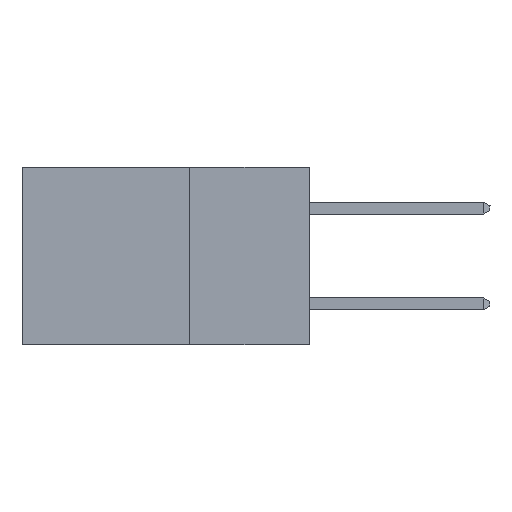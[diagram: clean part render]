
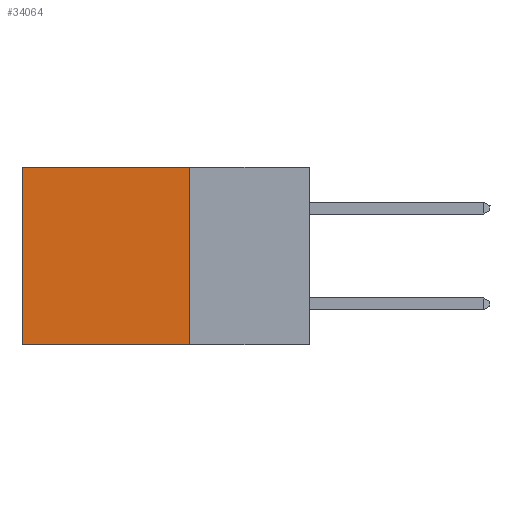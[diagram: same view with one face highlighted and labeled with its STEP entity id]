
A CAD part, left-side view. The second image highlights one B-rep face of the part: STEP entity #34064.
In plain terms, the highlighted planar face has unit normal (-1, 0, 0).
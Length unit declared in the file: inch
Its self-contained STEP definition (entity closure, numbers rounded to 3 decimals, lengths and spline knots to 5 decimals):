
#1798 = CARTESIAN_POINT ( 'NONE',  ( 0.2875, 0.25, 0. ) ) ;
#3241 = DIRECTION ( 'NONE',  ( 0., 0., -1. ) ) ;
#6987 = CARTESIAN_POINT ( 'NONE',  ( 0.2875, 0.25, -0.37 ) ) ;
#7099 = FACE_OUTER_BOUND ( 'NONE', #17099, .T. ) ;
#7116 = AXIS2_PLACEMENT_3D ( 'NONE', #1798, #23718, #32260 ) ;
#7215 = EDGE_CURVE ( 'NONE', #31215, #29491, #27271, .T. ) ;
#7290 = VECTOR ( 'NONE', #34912, 39.37008 ) ;
#8264 = LINE ( 'NONE', #27615, #22434 ) ;
#8357 = CARTESIAN_POINT ( 'NONE',  ( 0.2875, 0.6, 0. ) ) ;
#9704 = DIRECTION ( 'NONE',  ( 0., 0., -1. ) ) ;
#10205 = PLANE ( 'NONE',  #7116 ) ;
#10674 = CARTESIAN_POINT ( 'NONE',  ( 0.2875, 0.25, 0. ) ) ;
#10877 = CARTESIAN_POINT ( 'NONE',  ( 0.2875, 0.6, 0. ) ) ;
#11370 = LINE ( 'NONE', #20464, #34290 ) ;
#15477 = ORIENTED_EDGE ( 'NONE', *, *, #28930, .T. ) ;
#16179 = CARTESIAN_POINT ( 'NONE',  ( 0.2875, 0.6, -0.37 ) ) ;
#17099 = EDGE_LOOP ( 'NONE', ( #15477, #25730, #31753, #21285 ) ) ;
#18886 = EDGE_CURVE ( 'NONE', #31807, #20198, #8264, .T. ) ;
#20198 = VERTEX_POINT ( 'NONE', #16179 ) ;
#20464 = CARTESIAN_POINT ( 'NONE',  ( 0.2875, 0.25, 0. ) ) ;
#21285 = ORIENTED_EDGE ( 'NONE', *, *, #7215, .T. ) ;
#22434 = VECTOR ( 'NONE', #27258, 39.37008 ) ;
#22590 = LINE ( 'NONE', #8357, #22680 ) ;
#22680 = VECTOR ( 'NONE', #3241, 39.37008 ) ;
#23718 = DIRECTION ( 'NONE',  ( 1., 0., 0. ) ) ;
#24991 = CARTESIAN_POINT ( 'NONE',  ( 0.2875, 0.25, 0. ) ) ;
#25730 = ORIENTED_EDGE ( 'NONE', *, *, #18886, .F. ) ;
#27258 = DIRECTION ( 'NONE',  ( 0., 1., 0. ) ) ;
#27271 = LINE ( 'NONE', #10674, #7290 ) ;
#27615 = CARTESIAN_POINT ( 'NONE',  ( 0.2875, 0.25, -0.37 ) ) ;
#28154 = EDGE_CURVE ( 'NONE', #31215, #31807, #11370, .T. ) ;
#28930 = EDGE_CURVE ( 'NONE', #29491, #20198, #22590, .T. ) ;
#29491 = VERTEX_POINT ( 'NONE', #10877 ) ;
#31215 = VERTEX_POINT ( 'NONE', #24991 ) ;
#31753 = ORIENTED_EDGE ( 'NONE', *, *, #28154, .F. ) ;
#31807 = VERTEX_POINT ( 'NONE', #6987 ) ;
#32260 = DIRECTION ( 'NONE',  ( 0., 0., -1. ) ) ;
#34064 = ADVANCED_FACE ( 'NONE', ( #7099 ), #10205, .F. ) ;
#34290 = VECTOR ( 'NONE', #9704, 39.37008 ) ;
#34912 = DIRECTION ( 'NONE',  ( 0., 1., 0. ) ) ;
